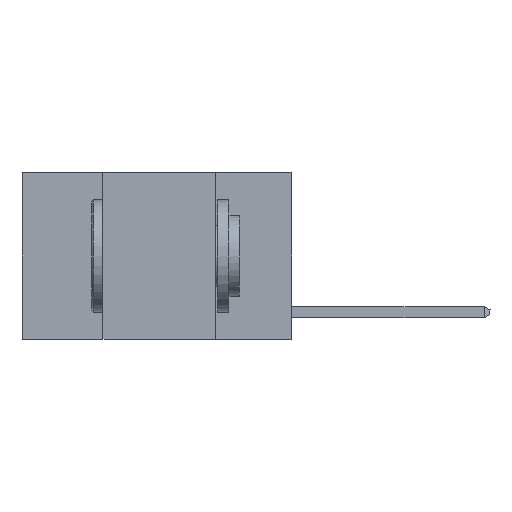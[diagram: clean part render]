
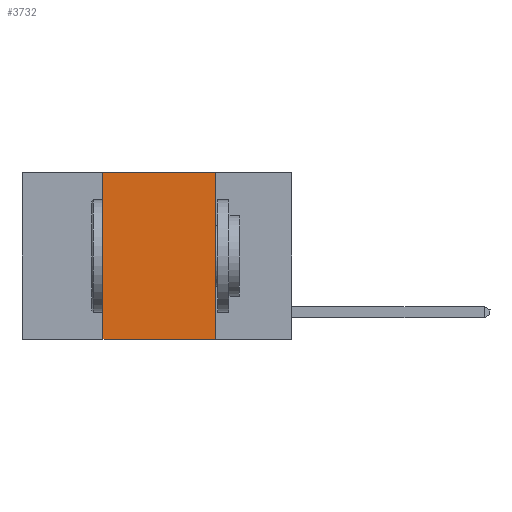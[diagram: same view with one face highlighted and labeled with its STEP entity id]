
A CAD part, left-side view. The second image highlights one B-rep face of the part: STEP entity #3732.
In plain terms, the highlighted planar face has unit normal (-1, 0, 0).
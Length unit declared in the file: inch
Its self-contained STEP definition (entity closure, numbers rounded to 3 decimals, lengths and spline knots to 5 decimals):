
#190 = DIRECTION ( 'NONE',  ( 0., 0., -1. ) ) ;
#337 = CARTESIAN_POINT ( 'NONE',  ( 0., 0.42, 0. ) ) ;
#1255 = EDGE_CURVE ( 'NONE', #16204, #4452, #3536, .T. ) ;
#1537 = CARTESIAN_POINT ( 'NONE',  ( 0., 0.17, 0. ) ) ;
#2174 = ORIENTED_EDGE ( 'NONE', *, *, #13402, .F. ) ;
#2734 = ORIENTED_EDGE ( 'NONE', *, *, #3831, .F. ) ;
#3251 = VECTOR ( 'NONE', #190, 39.37008 ) ;
#3442 = ORIENTED_EDGE ( 'NONE', *, *, #1255, .F. ) ;
#3536 = LINE ( 'NONE', #8927, #10410 ) ;
#3732 = ADVANCED_FACE ( 'NONE', ( #10492 ), #15935, .F. ) ;
#3831 = EDGE_CURVE ( 'NONE', #14418, #4685, #16290, .T. ) ;
#3966 = CARTESIAN_POINT ( 'NONE',  ( 0., 0.17, -0.37 ) ) ;
#4240 = LINE ( 'NONE', #14810, #6352 ) ;
#4452 = VERTEX_POINT ( 'NONE', #337 ) ;
#4685 = VERTEX_POINT ( 'NONE', #3966 ) ;
#6224 = CARTESIAN_POINT ( 'NONE',  ( 0., 0.6, 0. ) ) ;
#6352 = VECTOR ( 'NONE', #6882, 39.37008 ) ;
#6882 = DIRECTION ( 'NONE',  ( 0., -1., 0. ) ) ;
#7068 = LINE ( 'NONE', #10091, #7745 ) ;
#7635 = AXIS2_PLACEMENT_3D ( 'NONE', #6224, #9157, #13250 ) ;
#7745 = VECTOR ( 'NONE', #15544, 39.37008 ) ;
#8927 = CARTESIAN_POINT ( 'NONE',  ( 0., 0.42, 0. ) ) ;
#9098 = DIRECTION ( 'NONE',  ( 0., 0., 1. ) ) ;
#9157 = DIRECTION ( 'NONE',  ( 1., 0., 0. ) ) ;
#9263 = CARTESIAN_POINT ( 'NONE',  ( 0., 0.42, -0.37 ) ) ;
#10091 = CARTESIAN_POINT ( 'NONE',  ( 0., 0.6, -0.37 ) ) ;
#10410 = VECTOR ( 'NONE', #9098, 39.37008 ) ;
#10492 = FACE_OUTER_BOUND ( 'NONE', #15322, .T. ) ;
#10523 = EDGE_CURVE ( 'NONE', #16204, #4685, #7068, .T. ) ;
#13250 = DIRECTION ( 'NONE',  ( 0., 0., -1. ) ) ;
#13325 = CARTESIAN_POINT ( 'NONE',  ( 0., 0.17, 0. ) ) ;
#13402 = EDGE_CURVE ( 'NONE', #4452, #14418, #4240, .T. ) ;
#13978 = ORIENTED_EDGE ( 'NONE', *, *, #10523, .T. ) ;
#14418 = VERTEX_POINT ( 'NONE', #1537 ) ;
#14810 = CARTESIAN_POINT ( 'NONE',  ( 0., 0.6, 0. ) ) ;
#15322 = EDGE_LOOP ( 'NONE', ( #2734, #2174, #3442, #13978 ) ) ;
#15544 = DIRECTION ( 'NONE',  ( 0., -1., 0. ) ) ;
#15935 = PLANE ( 'NONE',  #7635 ) ;
#16204 = VERTEX_POINT ( 'NONE', #9263 ) ;
#16290 = LINE ( 'NONE', #13325, #3251 ) ;
